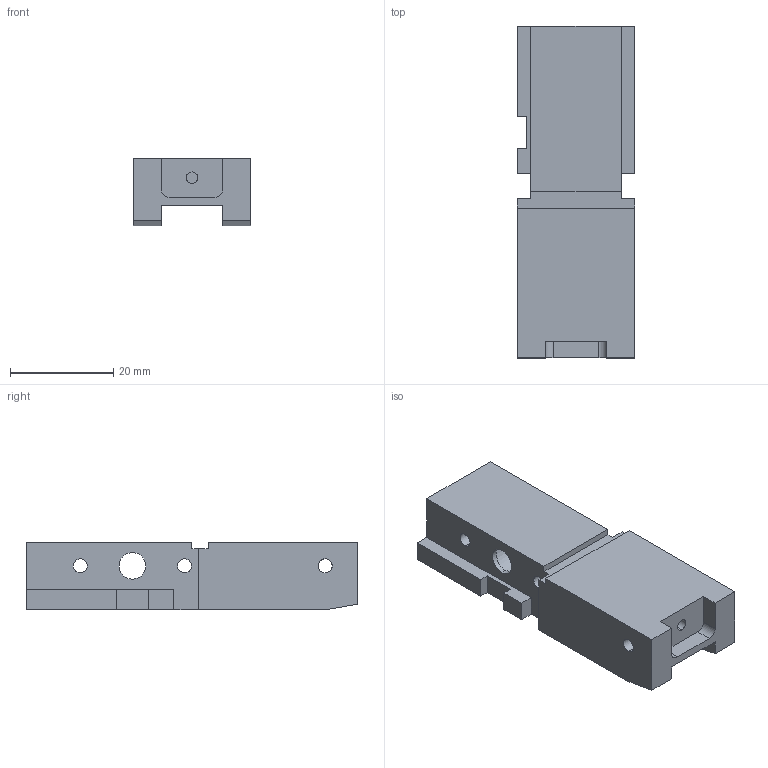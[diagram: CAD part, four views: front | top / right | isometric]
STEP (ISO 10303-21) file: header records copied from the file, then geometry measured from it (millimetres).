
FILE_DESCRIPTION (( 'STEP AP214' ), '1' );
FILE_NAME ('Original_Mag_Well_Rear.step', '2015-06-12T14:17:00', ( '' ), ( '' ), 'SwSTEP 2.0', 'SolidWorks 2015', '' );
FILE_SCHEMA (( 'AUTOMOTIVE_DESIGN' ));
Length unit declared in the file: inch
Products named in the file (1): Original_Mag_Well_Rear
Bounding box: 22.81 x 64.36 x 13.13 mm (x, y, z)
Volume: 12429.6 mm3; surface area: 6700.1 mm2
Topology: 1 solids, 1 shells, 56 faces, 158 edges, 104 vertices
Faces by surface type: plane 40, cylinder 16
Entity records: 1922 total; most frequent: CARTESIAN_POINT 387, ORIENTED_EDGE 316, DIRECTION 300, EDGE_CURVE 158, VECTOR 122, LINE 122, VERTEX_POINT 104, AXIS2_PLACEMENT_3D 89
